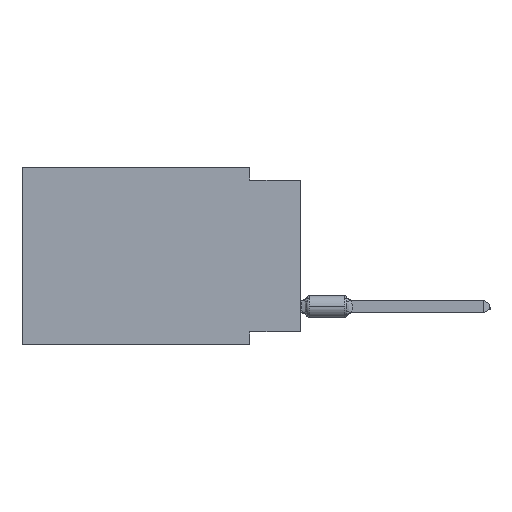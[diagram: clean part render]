
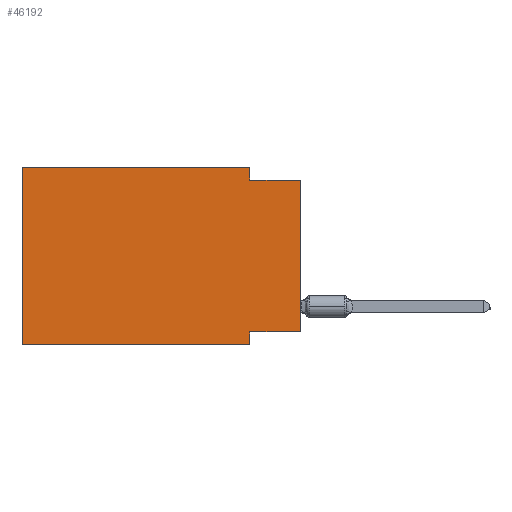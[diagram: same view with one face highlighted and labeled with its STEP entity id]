
A CAD part, left-side view. The second image highlights one B-rep face of the part: STEP entity #46192.
In plain terms, the highlighted planar face has unit normal (-1, 0, 0).
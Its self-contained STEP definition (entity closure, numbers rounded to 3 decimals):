
#704 = ORIENTED_EDGE ( 'NONE', *, *, #32452, .F. ) ;
#1932 = CARTESIAN_POINT ( 'NONE',  ( 0., 0., -8.255 ) ) ;
#2932 = VECTOR ( 'NONE', #37329, 1000. ) ;
#3375 = ORIENTED_EDGE ( 'NONE', *, *, #32626, .T. ) ;
#4080 = VERTEX_POINT ( 'NONE', #45859 ) ;
#4266 = VERTEX_POINT ( 'NONE', #31427 ) ;
#4350 = LINE ( 'NONE', #33063, #25985 ) ;
#4372 = LINE ( 'NONE', #42330, #14180 ) ;
#5103 = EDGE_CURVE ( 'NONE', #40540, #4266, #50181, .T. ) ;
#5318 = VECTOR ( 'NONE', #51814, 1000. ) ;
#6154 = FACE_OUTER_BOUND ( 'NONE', #38112, .T. ) ;
#6469 = CARTESIAN_POINT ( 'NONE',  ( 0., 13.97, -8.89 ) ) ;
#7901 = CARTESIAN_POINT ( 'NONE',  ( 0., 0., -8.255 ) ) ;
#8275 = VERTEX_POINT ( 'NONE', #33752 ) ;
#8702 = DIRECTION ( 'NONE',  ( 0., -1., 0. ) ) ;
#9282 = ORIENTED_EDGE ( 'NONE', *, *, #13106, .F. ) ;
#13106 = EDGE_CURVE ( 'NONE', #29759, #4080, #4350, .T. ) ;
#14180 = VECTOR ( 'NONE', #8702, 1000. ) ;
#14300 = CARTESIAN_POINT ( 'NONE',  ( 0., 13.97, 0. ) ) ;
#15518 = VERTEX_POINT ( 'NONE', #14300 ) ;
#15898 = ORIENTED_EDGE ( 'NONE', *, *, #35216, .F. ) ;
#17257 = CARTESIAN_POINT ( 'NONE',  ( 0., 0., -0.635 ) ) ;
#17478 = CARTESIAN_POINT ( 'NONE',  ( 0., 2.54, 0. ) ) ;
#17808 = AXIS2_PLACEMENT_3D ( 'NONE', #21827, #18319, #18064 ) ;
#18064 = DIRECTION ( 'NONE',  ( 0., 0., -1. ) ) ;
#18319 = DIRECTION ( 'NONE',  ( 1., 0., 0. ) ) ;
#21827 = CARTESIAN_POINT ( 'NONE',  ( 0., 13.97, 0. ) ) ;
#21831 = LINE ( 'NONE', #39192, #51936 ) ;
#23404 = EDGE_CURVE ( 'NONE', #4080, #27450, #29172, .T. ) ;
#25985 = VECTOR ( 'NONE', #49907, 1000. ) ;
#27450 = VERTEX_POINT ( 'NONE', #38920 ) ;
#27701 = EDGE_CURVE ( 'NONE', #4266, #8275, #33633, .T. ) ;
#28752 = ORIENTED_EDGE ( 'NONE', *, *, #27701, .F. ) ;
#29172 = LINE ( 'NONE', #17257, #2932 ) ;
#29759 = VERTEX_POINT ( 'NONE', #17478 ) ;
#30244 = DIRECTION ( 'NONE',  ( 0., 0., 1. ) ) ;
#30278 = ORIENTED_EDGE ( 'NONE', *, *, #30741, .T. ) ;
#30741 = EDGE_CURVE ( 'NONE', #35686, #8275, #51984, .T. ) ;
#31427 = CARTESIAN_POINT ( 'NONE',  ( 0., 2.54, -8.255 ) ) ;
#32040 = ORIENTED_EDGE ( 'NONE', *, *, #5103, .F. ) ;
#32452 = EDGE_CURVE ( 'NONE', #35686, #15518, #42900, .T. ) ;
#32626 = EDGE_CURVE ( 'NONE', #40540, #27450, #21831, .T. ) ;
#33063 = CARTESIAN_POINT ( 'NONE',  ( 0., 2.54, 0. ) ) ;
#33633 = LINE ( 'NONE', #42609, #43847 ) ;
#33752 = CARTESIAN_POINT ( 'NONE',  ( 0., 2.54, -8.89 ) ) ;
#35216 = EDGE_CURVE ( 'NONE', #15518, #29759, #4372, .T. ) ;
#35686 = VERTEX_POINT ( 'NONE', #6469 ) ;
#37329 = DIRECTION ( 'NONE',  ( 0., -1., 0. ) ) ;
#37416 = DIRECTION ( 'NONE',  ( 0., 1., 0. ) ) ;
#38112 = EDGE_LOOP ( 'NONE', ( #3375, #44837, #9282, #15898, #704, #30278, #28752, #32040 ) ) ;
#38407 = PLANE ( 'NONE',  #17808 ) ;
#38920 = CARTESIAN_POINT ( 'NONE',  ( 0., 0., -0.635 ) ) ;
#39192 = CARTESIAN_POINT ( 'NONE',  ( 0., 0., 0. ) ) ;
#39596 = CARTESIAN_POINT ( 'NONE',  ( 0., 13.97, 0. ) ) ;
#40540 = VERTEX_POINT ( 'NONE', #1932 ) ;
#40570 = DIRECTION ( 'NONE',  ( 0., -1., 0. ) ) ;
#40966 = VECTOR ( 'NONE', #37416, 1000. ) ;
#41054 = DIRECTION ( 'NONE',  ( 0., 0., -1. ) ) ;
#42330 = CARTESIAN_POINT ( 'NONE',  ( 0., 13.97, 0. ) ) ;
#42609 = CARTESIAN_POINT ( 'NONE',  ( 0., 2.54, -8.89 ) ) ;
#42900 = LINE ( 'NONE', #39596, #5318 ) ;
#43847 = VECTOR ( 'NONE', #41054, 1000. ) ;
#44837 = ORIENTED_EDGE ( 'NONE', *, *, #23404, .F. ) ;
#45859 = CARTESIAN_POINT ( 'NONE',  ( 0., 2.54, -0.635 ) ) ;
#46192 = ADVANCED_FACE ( 'NONE', ( #6154 ), #38407, .F. ) ;
#48452 = CARTESIAN_POINT ( 'NONE',  ( 0., 13.97, -8.89 ) ) ;
#49907 = DIRECTION ( 'NONE',  ( 0., 0., -1. ) ) ;
#50181 = LINE ( 'NONE', #7901, #40966 ) ;
#51814 = DIRECTION ( 'NONE',  ( 0., 0., 1. ) ) ;
#51936 = VECTOR ( 'NONE', #30244, 1000. ) ;
#51984 = LINE ( 'NONE', #48452, #52693 ) ;
#52693 = VECTOR ( 'NONE', #40570, 1000. ) ;
